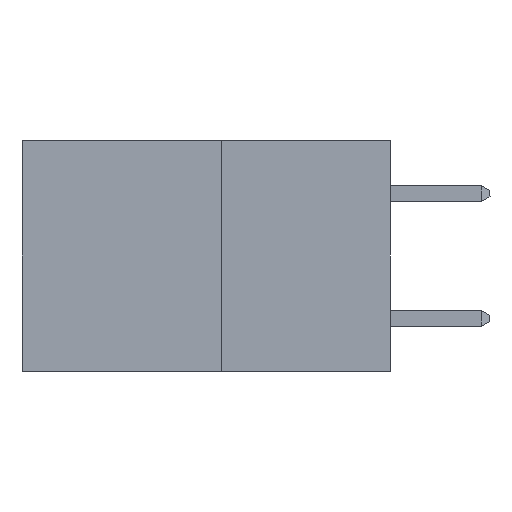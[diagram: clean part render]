
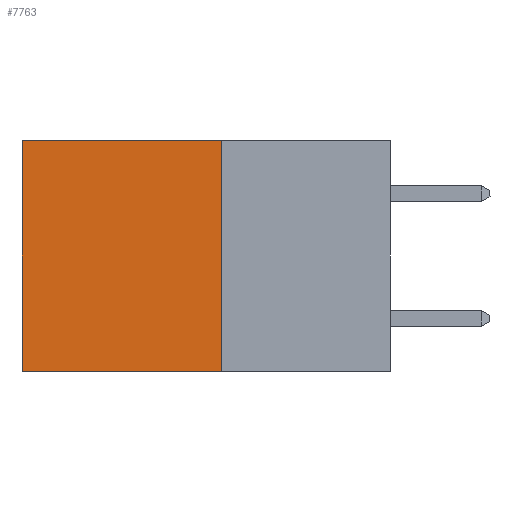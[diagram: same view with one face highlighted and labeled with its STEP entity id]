
A CAD part, left-side view. The second image highlights one B-rep face of the part: STEP entity #7763.
In plain terms, the highlighted planar face has unit normal (-1, 0, 0).
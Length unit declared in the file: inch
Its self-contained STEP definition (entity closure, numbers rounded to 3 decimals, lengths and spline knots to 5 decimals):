
#72 = VECTOR ( 'NONE', #981, 39.37008 ) ;
#167 = DIRECTION ( 'NONE',  ( 0., 0., -1. ) ) ;
#385 = ORIENTED_EDGE ( 'NONE', *, *, #6277, .T. ) ;
#408 = CARTESIAN_POINT ( 'NONE',  ( 0.277, 0.27, -0.37 ) ) ;
#525 = LINE ( 'NONE', #8129, #4301 ) ;
#601 = ORIENTED_EDGE ( 'NONE', *, *, #5887, .F. ) ;
#625 = DIRECTION ( 'NONE',  ( 0., 0., -1. ) ) ;
#702 = EDGE_CURVE ( 'NONE', #1745, #6395, #525, .T. ) ;
#826 = ORIENTED_EDGE ( 'NONE', *, *, #702, .T. ) ;
#981 = DIRECTION ( 'NONE',  ( 0., 0., -1. ) ) ;
#1096 = VECTOR ( 'NONE', #6077, 39.37008 ) ;
#1159 = CARTESIAN_POINT ( 'NONE',  ( 0.277, 0.59, 0. ) ) ;
#1745 = VERTEX_POINT ( 'NONE', #8099 ) ;
#2477 = ORIENTED_EDGE ( 'NONE', *, *, #7544, .F. ) ;
#3298 = CARTESIAN_POINT ( 'NONE',  ( 0.277, 0.27, -0.37 ) ) ;
#3341 = CARTESIAN_POINT ( 'NONE',  ( 0.277, 0.59, -0.37 ) ) ;
#3511 = VERTEX_POINT ( 'NONE', #3341 ) ;
#3729 = FACE_OUTER_BOUND ( 'NONE', #7834, .T. ) ;
#4084 = LINE ( 'NONE', #7155, #5298 ) ;
#4301 = VECTOR ( 'NONE', #8282, 39.37008 ) ;
#4847 = CARTESIAN_POINT ( 'NONE',  ( 0.277, 0.27, -0.37 ) ) ;
#4876 = LINE ( 'NONE', #3298, #1096 ) ;
#4879 = DIRECTION ( 'NONE',  ( 1., 0., 0. ) ) ;
#5195 = VERTEX_POINT ( 'NONE', #408 ) ;
#5298 = VECTOR ( 'NONE', #167, 39.37008 ) ;
#5887 = EDGE_CURVE ( 'NONE', #5195, #3511, #4876, .T. ) ;
#5910 = CARTESIAN_POINT ( 'NONE',  ( 0.277, 0.27, -0.37 ) ) ;
#6077 = DIRECTION ( 'NONE',  ( 0., 1., 0. ) ) ;
#6277 = EDGE_CURVE ( 'NONE', #6395, #3511, #4084, .T. ) ;
#6395 = VERTEX_POINT ( 'NONE', #1159 ) ;
#6803 = AXIS2_PLACEMENT_3D ( 'NONE', #4847, #4879, #625 ) ;
#7155 = CARTESIAN_POINT ( 'NONE',  ( 0.277, 0.59, -0.37 ) ) ;
#7544 = EDGE_CURVE ( 'NONE', #1745, #5195, #7715, .T. ) ;
#7715 = LINE ( 'NONE', #5910, #72 ) ;
#7763 = ADVANCED_FACE ( 'NONE', ( #3729 ), #8885, .F. ) ;
#7834 = EDGE_LOOP ( 'NONE', ( #385, #601, #2477, #826 ) ) ;
#8099 = CARTESIAN_POINT ( 'NONE',  ( 0.277, 0.27, 0. ) ) ;
#8129 = CARTESIAN_POINT ( 'NONE',  ( 0.277, 0.27, 0. ) ) ;
#8282 = DIRECTION ( 'NONE',  ( 0., 1., 0. ) ) ;
#8885 = PLANE ( 'NONE',  #6803 ) ;
